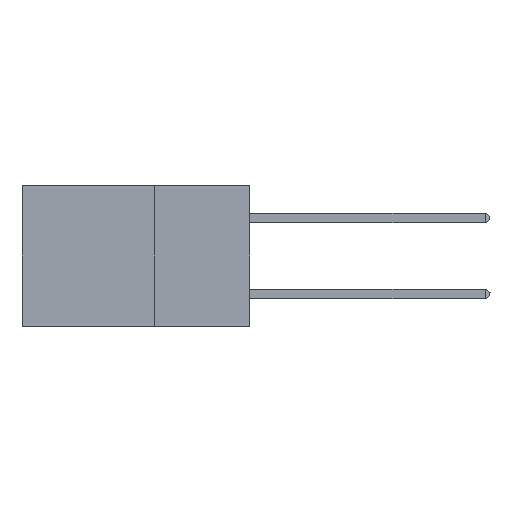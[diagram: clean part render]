
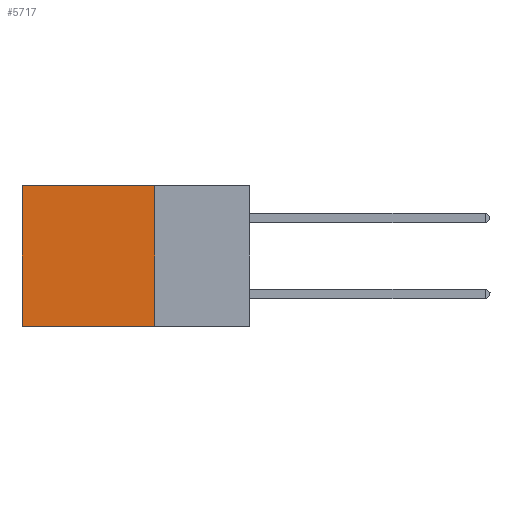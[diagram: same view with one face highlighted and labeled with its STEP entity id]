
A CAD part, left-side view. The second image highlights one B-rep face of the part: STEP entity #5717.
In plain terms, the highlighted planar face has unit normal (-1, 0, 0).
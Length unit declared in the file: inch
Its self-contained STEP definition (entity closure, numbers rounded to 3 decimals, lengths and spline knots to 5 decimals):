
#1267 = DIRECTION ( 'NONE',  ( 0., 0., -1. ) ) ;
#1627 = CARTESIAN_POINT ( 'NONE',  ( 0.2875, 0.6, 0. ) ) ;
#2701 = VECTOR ( 'NONE', #4952, 39.37008 ) ;
#3104 = EDGE_CURVE ( 'NONE', #13122, #14813, #10904, .T. ) ;
#4952 = DIRECTION ( 'NONE',  ( 0., 1., 0. ) ) ;
#5371 = EDGE_CURVE ( 'NONE', #9422, #14813, #7706, .T. ) ;
#5717 = ADVANCED_FACE ( 'NONE', ( #11757 ), #16687, .F. ) ;
#5932 = EDGE_LOOP ( 'NONE', ( #7601, #10526, #15812, #10152 ) ) ;
#6450 = DIRECTION ( 'NONE',  ( 0., 1., 0. ) ) ;
#6735 = CARTESIAN_POINT ( 'NONE',  ( 0.2875, 0.25, 0. ) ) ;
#6848 = CARTESIAN_POINT ( 'NONE',  ( 0.2875, 0.25, -0.37 ) ) ;
#7600 = VECTOR ( 'NONE', #6450, 39.37008 ) ;
#7601 = ORIENTED_EDGE ( 'NONE', *, *, #5371, .T. ) ;
#7706 = LINE ( 'NONE', #1627, #14345 ) ;
#7984 = CARTESIAN_POINT ( 'NONE',  ( 0.2875, 0.25, -0.37 ) ) ;
#9370 = CARTESIAN_POINT ( 'NONE',  ( 0.2875, 0.6, -0.37 ) ) ;
#9422 = VERTEX_POINT ( 'NONE', #12420 ) ;
#9733 = VECTOR ( 'NONE', #11264, 39.37008 ) ;
#9973 = CARTESIAN_POINT ( 'NONE',  ( 0.2875, 0.25, 0. ) ) ;
#10152 = ORIENTED_EDGE ( 'NONE', *, *, #14483, .T. ) ;
#10526 = ORIENTED_EDGE ( 'NONE', *, *, #3104, .F. ) ;
#10904 = LINE ( 'NONE', #7984, #7600 ) ;
#11102 = CARTESIAN_POINT ( 'NONE',  ( 0.2875, 0.25, 0. ) ) ;
#11264 = DIRECTION ( 'NONE',  ( 0., 0., -1. ) ) ;
#11757 = FACE_OUTER_BOUND ( 'NONE', #5932, .T. ) ;
#12092 = DIRECTION ( 'NONE',  ( 0., 0., -1. ) ) ;
#12420 = CARTESIAN_POINT ( 'NONE',  ( 0.2875, 0.6, 0. ) ) ;
#13043 = LINE ( 'NONE', #9973, #9733 ) ;
#13122 = VERTEX_POINT ( 'NONE', #6848 ) ;
#14221 = DIRECTION ( 'NONE',  ( 1., 0., 0. ) ) ;
#14345 = VECTOR ( 'NONE', #12092, 39.37008 ) ;
#14461 = EDGE_CURVE ( 'NONE', #15481, #13122, #13043, .T. ) ;
#14483 = EDGE_CURVE ( 'NONE', #15481, #9422, #16349, .T. ) ;
#14813 = VERTEX_POINT ( 'NONE', #9370 ) ;
#14905 = AXIS2_PLACEMENT_3D ( 'NONE', #6735, #14221, #1267 ) ;
#15481 = VERTEX_POINT ( 'NONE', #11102 ) ;
#15812 = ORIENTED_EDGE ( 'NONE', *, *, #14461, .F. ) ;
#16236 = CARTESIAN_POINT ( 'NONE',  ( 0.2875, 0.25, 0. ) ) ;
#16349 = LINE ( 'NONE', #16236, #2701 ) ;
#16687 = PLANE ( 'NONE',  #14905 ) ;
